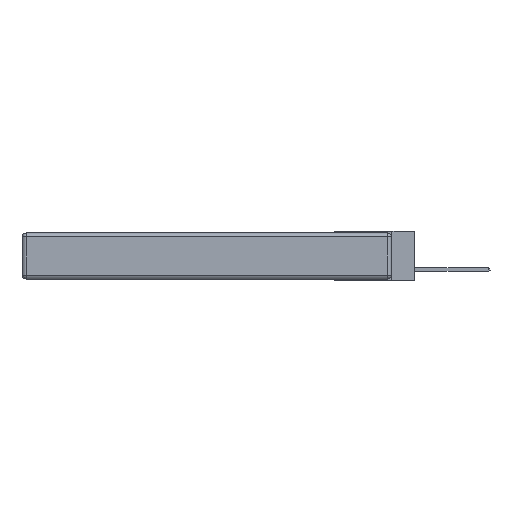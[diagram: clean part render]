
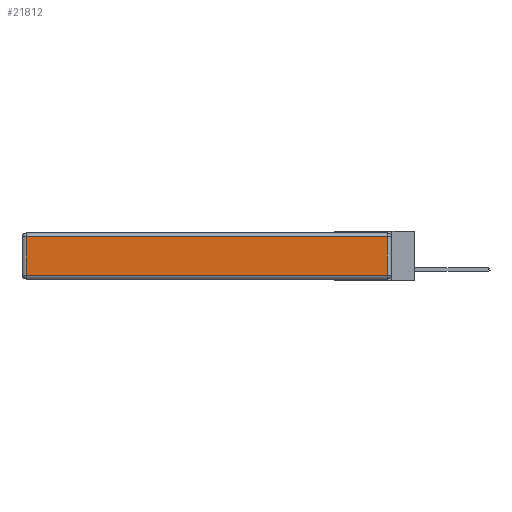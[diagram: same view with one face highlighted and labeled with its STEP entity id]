
A CAD part, left-side view. The second image highlights one B-rep face of the part: STEP entity #21812.
In plain terms, the highlighted planar face has unit normal (-1, 0, 0).
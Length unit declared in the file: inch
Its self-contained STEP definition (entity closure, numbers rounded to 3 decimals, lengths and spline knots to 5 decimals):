
#313 = DIRECTION ( 'NONE',  ( 0., 1., 0. ) ) ;
#422 = VECTOR ( 'NONE', #27753, 39.37008 ) ;
#703 = EDGE_CURVE ( 'NONE', #5045, #13792, #32613, .T. ) ;
#1471 = ORIENTED_EDGE ( 'NONE', *, *, #703, .T. ) ;
#1665 = VERTEX_POINT ( 'NONE', #16958 ) ;
#2198 = CARTESIAN_POINT ( 'NONE',  ( 0., 2.72, -0.313 ) ) ;
#2988 = LINE ( 'NONE', #10989, #10525 ) ;
#3191 = CARTESIAN_POINT ( 'NONE',  ( 0., 2.75, -0.03 ) ) ;
#4300 = ORIENTED_EDGE ( 'NONE', *, *, #26423, .T. ) ;
#4756 = CARTESIAN_POINT ( 'NONE',  ( 0., 2.72, -0.343 ) ) ;
#5045 = VERTEX_POINT ( 'NONE', #17864 ) ;
#5226 = DIRECTION ( 'NONE',  ( 0., -1., 0. ) ) ;
#6594 = DIRECTION ( 'NONE',  ( 0., 0., 1. ) ) ;
#9037 = EDGE_LOOP ( 'NONE', ( #23715, #4300, #11888, #1471 ) ) ;
#9368 = VECTOR ( 'NONE', #313, 39.37008 ) ;
#10525 = VECTOR ( 'NONE', #5226, 39.37008 ) ;
#10989 = CARTESIAN_POINT ( 'NONE',  ( 0., 0., -0.313 ) ) ;
#11888 = ORIENTED_EDGE ( 'NONE', *, *, #32475, .T. ) ;
#13792 = VERTEX_POINT ( 'NONE', #2198 ) ;
#14702 = LINE ( 'NONE', #14753, #17902 ) ;
#14753 = CARTESIAN_POINT ( 'NONE',  ( 0., 0.03, -0.343 ) ) ;
#16785 = PLANE ( 'NONE',  #20307 ) ;
#16958 = CARTESIAN_POINT ( 'NONE',  ( 0., 0.03, -0.313 ) ) ;
#17129 = VERTEX_POINT ( 'NONE', #26123 ) ;
#17864 = CARTESIAN_POINT ( 'NONE',  ( 0., 2.72, -0.03 ) ) ;
#17902 = VECTOR ( 'NONE', #6594, 39.37008 ) ;
#19992 = FACE_OUTER_BOUND ( 'NONE', #9037, .T. ) ;
#20307 = AXIS2_PLACEMENT_3D ( 'NONE', #26982, #21638, #29620 ) ;
#20601 = EDGE_CURVE ( 'NONE', #13792, #1665, #2988, .T. ) ;
#21638 = DIRECTION ( 'NONE',  ( -1., 0., 0. ) ) ;
#21812 = ADVANCED_FACE ( 'NONE', ( #19992 ), #16785, .T. ) ;
#23715 = ORIENTED_EDGE ( 'NONE', *, *, #20601, .T. ) ;
#26123 = CARTESIAN_POINT ( 'NONE',  ( 0., 0.03, -0.03 ) ) ;
#26423 = EDGE_CURVE ( 'NONE', #1665, #17129, #14702, .T. ) ;
#26982 = CARTESIAN_POINT ( 'NONE',  ( 0., 0., -0.343 ) ) ;
#27753 = DIRECTION ( 'NONE',  ( 0., 0., -1. ) ) ;
#29620 = DIRECTION ( 'NONE',  ( 0., 0., 1. ) ) ;
#32408 = LINE ( 'NONE', #3191, #9368 ) ;
#32475 = EDGE_CURVE ( 'NONE', #17129, #5045, #32408, .T. ) ;
#32613 = LINE ( 'NONE', #4756, #422 ) ;
